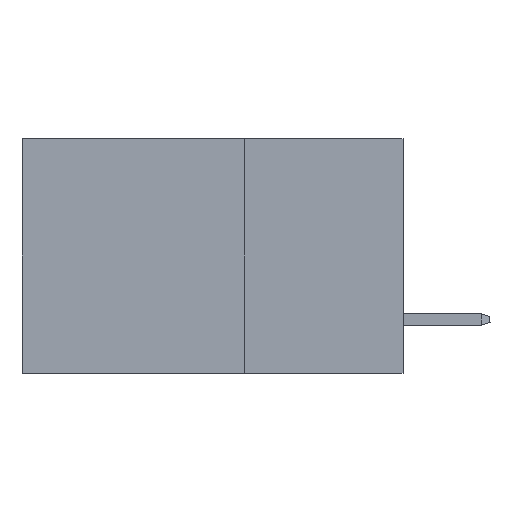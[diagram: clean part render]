
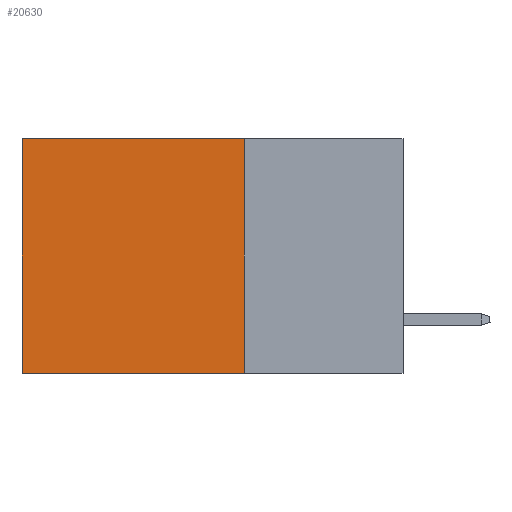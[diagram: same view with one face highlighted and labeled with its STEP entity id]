
A CAD part, left-side view. The second image highlights one B-rep face of the part: STEP entity #20630.
In plain terms, the highlighted planar face has unit normal (-1, 0, 0).
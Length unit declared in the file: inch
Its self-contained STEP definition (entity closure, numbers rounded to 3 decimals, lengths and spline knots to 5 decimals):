
#459 = CARTESIAN_POINT ( 'NONE',  ( 0.2875, 0.6, 0. ) ) ;
#874 = EDGE_LOOP ( 'NONE', ( #14190, #15878, #21135, #8727 ) ) ;
#1436 = DIRECTION ( 'NONE',  ( 0., 0., -1. ) ) ;
#1885 = EDGE_CURVE ( 'NONE', #16792, #12099, #20202, .T. ) ;
#3503 = VECTOR ( 'NONE', #22342, 39.37008 ) ;
#3666 = VERTEX_POINT ( 'NONE', #35797 ) ;
#4797 = CARTESIAN_POINT ( 'NONE',  ( 0.2875, 0.25, 0. ) ) ;
#4969 = CARTESIAN_POINT ( 'NONE',  ( 0.2875, 0.25, -0.37 ) ) ;
#7331 = CARTESIAN_POINT ( 'NONE',  ( 0.2875, 0.6, -0.37 ) ) ;
#7373 = DIRECTION ( 'NONE',  ( 1., 0., 0. ) ) ;
#8727 = ORIENTED_EDGE ( 'NONE', *, *, #9087, .T. ) ;
#9087 = EDGE_CURVE ( 'NONE', #3666, #16792, #20617, .T. ) ;
#10540 = FACE_OUTER_BOUND ( 'NONE', #874, .T. ) ;
#10855 = CARTESIAN_POINT ( 'NONE',  ( 0.2875, 0.25, -0.37 ) ) ;
#11598 = CARTESIAN_POINT ( 'NONE',  ( 0.2875, 0.25, 0. ) ) ;
#12099 = VERTEX_POINT ( 'NONE', #7331 ) ;
#14190 = ORIENTED_EDGE ( 'NONE', *, *, #1885, .T. ) ;
#15878 = ORIENTED_EDGE ( 'NONE', *, *, #21100, .F. ) ;
#16384 = PLANE ( 'NONE',  #28043 ) ;
#16746 = CARTESIAN_POINT ( 'NONE',  ( 0.2875, 0.25, 0. ) ) ;
#16792 = VERTEX_POINT ( 'NONE', #32549 ) ;
#20202 = LINE ( 'NONE', #459, #34948 ) ;
#20617 = LINE ( 'NONE', #11598, #22085 ) ;
#20630 = ADVANCED_FACE ( 'NONE', ( #10540 ), #16384, .F. ) ;
#21100 = EDGE_CURVE ( 'NONE', #29807, #12099, #25184, .T. ) ;
#21135 = ORIENTED_EDGE ( 'NONE', *, *, #25260, .F. ) ;
#22085 = VECTOR ( 'NONE', #23429, 39.37008 ) ;
#22342 = DIRECTION ( 'NONE',  ( 0., 1., 0. ) ) ;
#23429 = DIRECTION ( 'NONE',  ( 0., 1., 0. ) ) ;
#25184 = LINE ( 'NONE', #10855, #3503 ) ;
#25260 = EDGE_CURVE ( 'NONE', #3666, #29807, #30616, .T. ) ;
#28043 = AXIS2_PLACEMENT_3D ( 'NONE', #16746, #7373, #36513 ) ;
#29246 = DIRECTION ( 'NONE',  ( 0., 0., -1. ) ) ;
#29807 = VERTEX_POINT ( 'NONE', #4969 ) ;
#30616 = LINE ( 'NONE', #4797, #36105 ) ;
#32549 = CARTESIAN_POINT ( 'NONE',  ( 0.2875, 0.6, 0. ) ) ;
#34948 = VECTOR ( 'NONE', #29246, 39.37008 ) ;
#35797 = CARTESIAN_POINT ( 'NONE',  ( 0.2875, 0.25, 0. ) ) ;
#36105 = VECTOR ( 'NONE', #1436, 39.37008 ) ;
#36513 = DIRECTION ( 'NONE',  ( 0., 0., -1. ) ) ;
